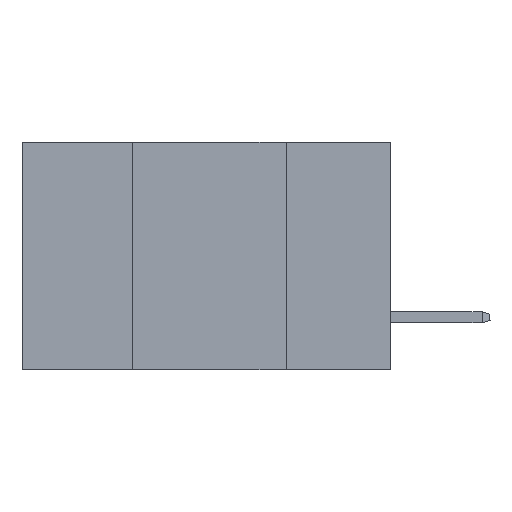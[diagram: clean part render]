
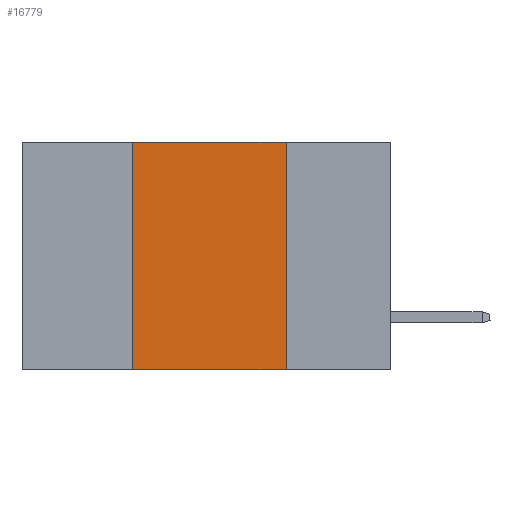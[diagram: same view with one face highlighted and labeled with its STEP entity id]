
A CAD part, left-side view. The second image highlights one B-rep face of the part: STEP entity #16779.
In plain terms, the highlighted planar face has unit normal (-1, 0, 0).
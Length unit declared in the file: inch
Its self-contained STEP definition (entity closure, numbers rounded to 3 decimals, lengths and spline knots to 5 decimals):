
#2773 = EDGE_CURVE ( 'NONE', #16652, #18207, #35868, .T. ) ;
#4188 = VECTOR ( 'NONE', #20690, 39.37008 ) ;
#5259 = VECTOR ( 'NONE', #6930, 39.37008 ) ;
#6339 = CARTESIAN_POINT ( 'NONE',  ( 0., 0.17, -0.37 ) ) ;
#6930 = DIRECTION ( 'NONE',  ( 0., -1., 0. ) ) ;
#7274 = CARTESIAN_POINT ( 'NONE',  ( 0., 0.6, 0. ) ) ;
#8261 = PLANE ( 'NONE',  #35653 ) ;
#10566 = CARTESIAN_POINT ( 'NONE',  ( 0., 0.42, 0. ) ) ;
#13122 = CARTESIAN_POINT ( 'NONE',  ( 0., 0.42, 0. ) ) ;
#13845 = ORIENTED_EDGE ( 'NONE', *, *, #20410, .F. ) ;
#15776 = ORIENTED_EDGE ( 'NONE', *, *, #33786, .T. ) ;
#16289 = EDGE_LOOP ( 'NONE', ( #18056, #26013, #13845, #15776 ) ) ;
#16652 = VERTEX_POINT ( 'NONE', #10566 ) ;
#16779 = ADVANCED_FACE ( 'NONE', ( #19699 ), #8261, .F. ) ;
#17478 = LINE ( 'NONE', #36324, #31521 ) ;
#17635 = DIRECTION ( 'NONE',  ( 1., 0., 0. ) ) ;
#17791 = CARTESIAN_POINT ( 'NONE',  ( 0., 0.6, 0. ) ) ;
#18056 = ORIENTED_EDGE ( 'NONE', *, *, #36513, .F. ) ;
#18207 = VERTEX_POINT ( 'NONE', #39283 ) ;
#19699 = FACE_OUTER_BOUND ( 'NONE', #16289, .T. ) ;
#20410 = EDGE_CURVE ( 'NONE', #35444, #16652, #25498, .T. ) ;
#20690 = DIRECTION ( 'NONE',  ( 0., -1., 0. ) ) ;
#21092 = DIRECTION ( 'NONE',  ( 0., 0., -1. ) ) ;
#25498 = LINE ( 'NONE', #13122, #38511 ) ;
#26013 = ORIENTED_EDGE ( 'NONE', *, *, #2773, .F. ) ;
#26598 = VERTEX_POINT ( 'NONE', #6339 ) ;
#26603 = DIRECTION ( 'NONE',  ( 0., 0., 1. ) ) ;
#29987 = CARTESIAN_POINT ( 'NONE',  ( 0., 0.6, -0.37 ) ) ;
#31521 = VECTOR ( 'NONE', #39904, 39.37008 ) ;
#33786 = EDGE_CURVE ( 'NONE', #35444, #26598, #35345, .T. ) ;
#35345 = LINE ( 'NONE', #29987, #5259 ) ;
#35444 = VERTEX_POINT ( 'NONE', #35535 ) ;
#35535 = CARTESIAN_POINT ( 'NONE',  ( 0., 0.42, -0.37 ) ) ;
#35653 = AXIS2_PLACEMENT_3D ( 'NONE', #17791, #17635, #21092 ) ;
#35868 = LINE ( 'NONE', #7274, #4188 ) ;
#36324 = CARTESIAN_POINT ( 'NONE',  ( 0., 0.17, 0. ) ) ;
#36513 = EDGE_CURVE ( 'NONE', #18207, #26598, #17478, .T. ) ;
#38511 = VECTOR ( 'NONE', #26603, 39.37008 ) ;
#39283 = CARTESIAN_POINT ( 'NONE',  ( 0., 0.17, 0. ) ) ;
#39904 = DIRECTION ( 'NONE',  ( 0., 0., -1. ) ) ;
